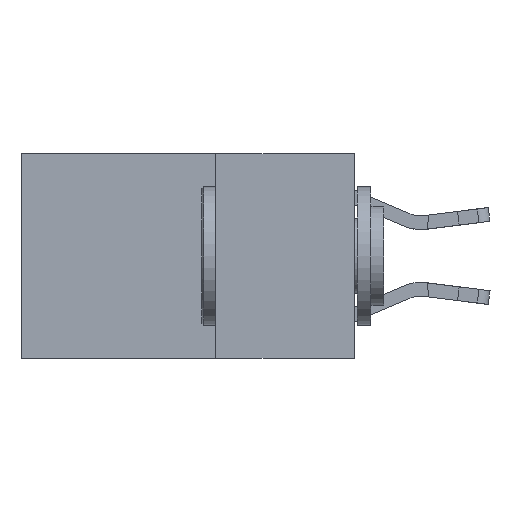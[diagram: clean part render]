
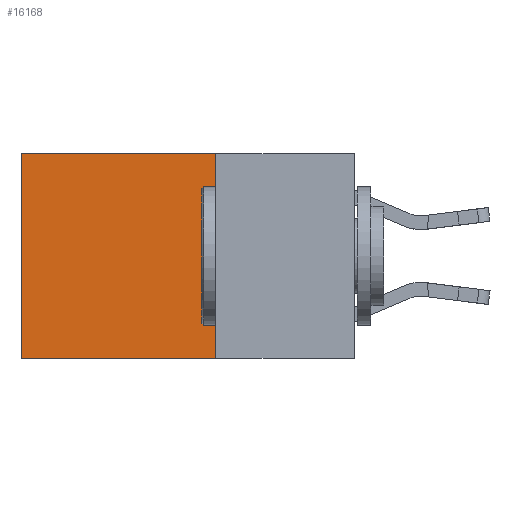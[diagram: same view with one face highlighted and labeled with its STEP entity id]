
A CAD part, left-side view. The second image highlights one B-rep face of the part: STEP entity #16168.
In plain terms, the highlighted planar face has unit normal (-1, 0, 0).
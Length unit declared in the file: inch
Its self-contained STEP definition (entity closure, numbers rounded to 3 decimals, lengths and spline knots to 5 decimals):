
#2 = AXIS2_PLACEMENT_3D ( 'NONE', #16695, #6488, #18391 ) ;
#1841 = DIRECTION ( 'NONE',  ( 0., 0., -1. ) ) ;
#2336 = EDGE_CURVE ( 'NONE', #8058, #8540, #4937, .T. ) ;
#3431 = DIRECTION ( 'NONE',  ( 0., 1., 0. ) ) ;
#4937 = LINE ( 'NONE', #13799, #17474 ) ;
#5002 = LINE ( 'NONE', #18797, #22088 ) ;
#5783 = VERTEX_POINT ( 'NONE', #11887 ) ;
#5837 = EDGE_CURVE ( 'NONE', #5783, #8058, #5002, .T. ) ;
#6488 = DIRECTION ( 'NONE',  ( 1., 0., 0. ) ) ;
#7461 = DIRECTION ( 'NONE',  ( 0., 0., -1. ) ) ;
#8058 = VERTEX_POINT ( 'NONE', #13898 ) ;
#8464 = VERTEX_POINT ( 'NONE', #18255 ) ;
#8540 = VERTEX_POINT ( 'NONE', #21857 ) ;
#9436 = LINE ( 'NONE', #19368, #17952 ) ;
#11540 = PLANE ( 'NONE',  #2 ) ;
#11887 = CARTESIAN_POINT ( 'NONE',  ( 0.2625, 0.25, 0. ) ) ;
#13799 = CARTESIAN_POINT ( 'NONE',  ( 0.2625, 0.6, 0. ) ) ;
#13898 = CARTESIAN_POINT ( 'NONE',  ( 0.2625, 0.6, 0. ) ) ;
#13949 = EDGE_CURVE ( 'NONE', #5783, #8464, #9436, .T. ) ;
#13990 = EDGE_LOOP ( 'NONE', ( #17550, #21212, #19054, #20616 ) ) ;
#15779 = EDGE_CURVE ( 'NONE', #8464, #8540, #20545, .T. ) ;
#16168 = ADVANCED_FACE ( 'NONE', ( #22145 ), #11540, .F. ) ;
#16695 = CARTESIAN_POINT ( 'NONE',  ( 0.2625, 0.25, 0. ) ) ;
#17474 = VECTOR ( 'NONE', #1841, 39.37008 ) ;
#17550 = ORIENTED_EDGE ( 'NONE', *, *, #2336, .T. ) ;
#17952 = VECTOR ( 'NONE', #7461, 39.37008 ) ;
#18255 = CARTESIAN_POINT ( 'NONE',  ( 0.2625, 0.25, -0.37 ) ) ;
#18391 = DIRECTION ( 'NONE',  ( 0., 0., -1. ) ) ;
#18797 = CARTESIAN_POINT ( 'NONE',  ( 0.2625, 0.25, 0. ) ) ;
#19054 = ORIENTED_EDGE ( 'NONE', *, *, #13949, .F. ) ;
#19368 = CARTESIAN_POINT ( 'NONE',  ( 0.2625, 0.25, 0. ) ) ;
#20531 = DIRECTION ( 'NONE',  ( 0., 1., 0. ) ) ;
#20545 = LINE ( 'NONE', #22152, #21075 ) ;
#20616 = ORIENTED_EDGE ( 'NONE', *, *, #5837, .T. ) ;
#21075 = VECTOR ( 'NONE', #3431, 39.37008 ) ;
#21212 = ORIENTED_EDGE ( 'NONE', *, *, #15779, .F. ) ;
#21857 = CARTESIAN_POINT ( 'NONE',  ( 0.2625, 0.6, -0.37 ) ) ;
#22088 = VECTOR ( 'NONE', #20531, 39.37008 ) ;
#22145 = FACE_OUTER_BOUND ( 'NONE', #13990, .T. ) ;
#22152 = CARTESIAN_POINT ( 'NONE',  ( 0.2625, 0.25, -0.37 ) ) ;
